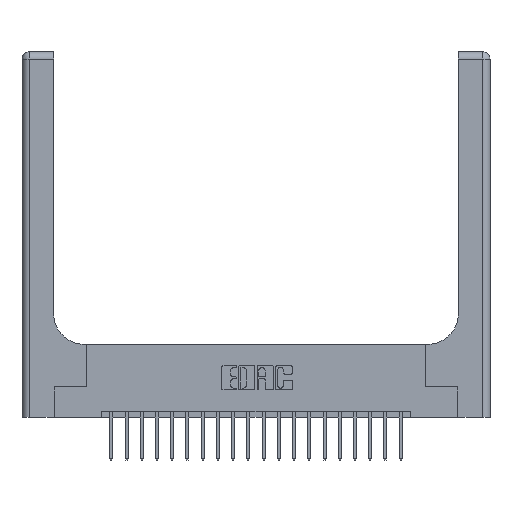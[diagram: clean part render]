
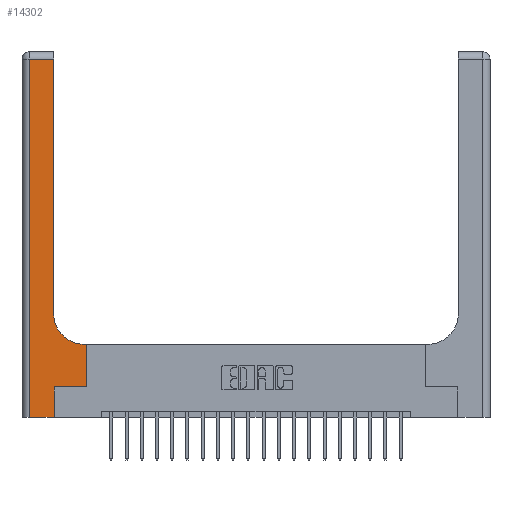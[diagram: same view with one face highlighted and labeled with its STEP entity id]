
A CAD part, top view. The second image highlights one B-rep face of the part: STEP entity #14302.
In plain terms, the highlighted planar face has unit normal (0, 0, 1).
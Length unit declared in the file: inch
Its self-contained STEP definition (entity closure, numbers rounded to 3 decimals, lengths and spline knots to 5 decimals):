
#877 = VECTOR ( 'NONE', #13834, 39.37008 ) ;
#1749 = CARTESIAN_POINT ( 'NONE',  ( 0.26, 0.85, 0.37 ) ) ;
#1812 = DIRECTION ( 'NONE',  ( 0., 1., 0. ) ) ;
#1875 = CARTESIAN_POINT ( 'NONE',  ( 0.265, 0.25, 0.37 ) ) ;
#2048 = CIRCLE ( 'NONE', #18115, 0.25 ) ;
#2377 = CARTESIAN_POINT ( 'NONE',  ( 0.26, 0.6, 0.37 ) ) ;
#2466 = VERTEX_POINT ( 'NONE', #2487 ) ;
#2487 = CARTESIAN_POINT ( 'NONE',  ( 0.528, 0.6, 0.37 ) ) ;
#2819 = FACE_OUTER_BOUND ( 'NONE', #20331, .T. ) ;
#3313 = EDGE_CURVE ( 'NONE', #4291, #10176, #8807, .T. ) ;
#3326 = CARTESIAN_POINT ( 'NONE',  ( 0.51, 0.85, 0.37 ) ) ;
#3874 = LINE ( 'NONE', #21223, #18756 ) ;
#4291 = VERTEX_POINT ( 'NONE', #5301 ) ;
#4418 = VECTOR ( 'NONE', #8481, 39.37008 ) ;
#4441 = CARTESIAN_POINT ( 'NONE',  ( 0.26, 3., 0.37 ) ) ;
#4511 = ORIENTED_EDGE ( 'NONE', *, *, #6771, .T. ) ;
#4532 = VERTEX_POINT ( 'NONE', #20675 ) ;
#5008 = CARTESIAN_POINT ( 'NONE',  ( 0.528, 0.25, 0.37 ) ) ;
#5301 = CARTESIAN_POINT ( 'NONE',  ( 0.26, 2.94, 0.37 ) ) ;
#5614 = CARTESIAN_POINT ( 'NONE',  ( 0.06, 2.94, 0.37 ) ) ;
#6077 = PLANE ( 'NONE',  #6587 ) ;
#6587 = AXIS2_PLACEMENT_3D ( 'NONE', #7767, #17749, #12679 ) ;
#6771 = EDGE_CURVE ( 'NONE', #4532, #15937, #3874, .T. ) ;
#6959 = VECTOR ( 'NONE', #1812, 39.37008 ) ;
#7087 = VECTOR ( 'NONE', #17855, 39.37008 ) ;
#7767 = CARTESIAN_POINT ( 'NONE',  ( 0., 3., 0.37 ) ) ;
#7911 = DIRECTION ( 'NONE',  ( 1., 0., 0. ) ) ;
#8481 = DIRECTION ( 'NONE',  ( -1., 0., 0. ) ) ;
#8807 = LINE ( 'NONE', #13137, #4418 ) ;
#8896 = EDGE_CURVE ( 'NONE', #13702, #12847, #14351, .T. ) ;
#9133 = CARTESIAN_POINT ( 'NONE',  ( 0.265, 0., 0.37 ) ) ;
#9296 = EDGE_CURVE ( 'NONE', #13428, #17896, #2048, .T. ) ;
#9628 = CARTESIAN_POINT ( 'NONE',  ( 0.528, 0.25, 0.37 ) ) ;
#9748 = ORIENTED_EDGE ( 'NONE', *, *, #19689, .T. ) ;
#10176 = VERTEX_POINT ( 'NONE', #5614 ) ;
#10810 = ORIENTED_EDGE ( 'NONE', *, *, #9296, .T. ) ;
#11851 = LINE ( 'NONE', #14989, #6959 ) ;
#11991 = DIRECTION ( 'NONE',  ( -1., 0., 0. ) ) ;
#11995 = EDGE_CURVE ( 'NONE', #2466, #13428, #14976, .T. ) ;
#12679 = DIRECTION ( 'NONE',  ( -1., 0., 0. ) ) ;
#12681 = LINE ( 'NONE', #20405, #877 ) ;
#12847 = VERTEX_POINT ( 'NONE', #5008 ) ;
#12922 = VECTOR ( 'NONE', #17853, 39.37008 ) ;
#13137 = CARTESIAN_POINT ( 'NONE',  ( 0., 2.94, 0.37 ) ) ;
#13422 = ORIENTED_EDGE ( 'NONE', *, *, #3313, .T. ) ;
#13428 = VERTEX_POINT ( 'NONE', #18912 ) ;
#13507 = LINE ( 'NONE', #9628, #7087 ) ;
#13702 = VERTEX_POINT ( 'NONE', #18684 ) ;
#13834 = DIRECTION ( 'NONE',  ( 0., -1., 0. ) ) ;
#14302 = ADVANCED_FACE ( 'NONE', ( #2819 ), #6077, .F. ) ;
#14351 = LINE ( 'NONE', #1875, #18186 ) ;
#14806 = DIRECTION ( 'NONE',  ( 0., 0., -1. ) ) ;
#14976 = LINE ( 'NONE', #2377, #19041 ) ;
#14989 = CARTESIAN_POINT ( 'NONE',  ( 0.265, 0., 0.37 ) ) ;
#15937 = VERTEX_POINT ( 'NONE', #9133 ) ;
#16009 = EDGE_CURVE ( 'NONE', #12847, #2466, #13507, .T. ) ;
#16020 = ORIENTED_EDGE ( 'NONE', *, *, #8896, .T. ) ;
#16616 = ORIENTED_EDGE ( 'NONE', *, *, #21149, .T. ) ;
#17623 = EDGE_CURVE ( 'NONE', #17896, #4291, #18338, .T. ) ;
#17749 = DIRECTION ( 'NONE',  ( 0., 0., -1. ) ) ;
#17853 = DIRECTION ( 'NONE',  ( 0., 1., 0. ) ) ;
#17855 = DIRECTION ( 'NONE',  ( 0., 1., 0. ) ) ;
#17896 = VERTEX_POINT ( 'NONE', #1749 ) ;
#17919 = ORIENTED_EDGE ( 'NONE', *, *, #17623, .T. ) ;
#18115 = AXIS2_PLACEMENT_3D ( 'NONE', #3326, #14806, #19731 ) ;
#18186 = VECTOR ( 'NONE', #18806, 39.37008 ) ;
#18338 = LINE ( 'NONE', #4441, #12922 ) ;
#18684 = CARTESIAN_POINT ( 'NONE',  ( 0.265, 0.25, 0.37 ) ) ;
#18756 = VECTOR ( 'NONE', #7911, 39.37008 ) ;
#18806 = DIRECTION ( 'NONE',  ( 1., 0., 0. ) ) ;
#18912 = CARTESIAN_POINT ( 'NONE',  ( 0.51, 0.6, 0.37 ) ) ;
#19041 = VECTOR ( 'NONE', #11991, 39.37008 ) ;
#19159 = ORIENTED_EDGE ( 'NONE', *, *, #11995, .T. ) ;
#19689 = EDGE_CURVE ( 'NONE', #10176, #4532, #12681, .T. ) ;
#19731 = DIRECTION ( 'NONE',  ( 1., 0., 0. ) ) ;
#20106 = ORIENTED_EDGE ( 'NONE', *, *, #16009, .T. ) ;
#20331 = EDGE_LOOP ( 'NONE', ( #17919, #13422, #9748, #4511, #16616, #16020, #20106, #19159, #10810 ) ) ;
#20405 = CARTESIAN_POINT ( 'NONE',  ( 0.06, 3., 0.37 ) ) ;
#20675 = CARTESIAN_POINT ( 'NONE',  ( 0.06, 0., 0.37 ) ) ;
#21149 = EDGE_CURVE ( 'NONE', #15937, #13702, #11851, .T. ) ;
#21223 = CARTESIAN_POINT ( 'NONE',  ( 0., 0., 0.37 ) ) ;
